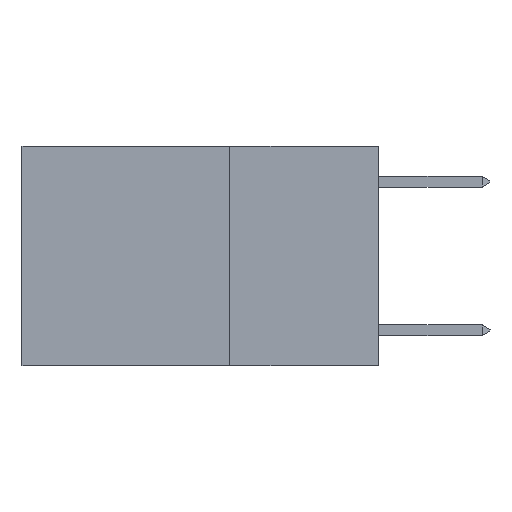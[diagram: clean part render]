
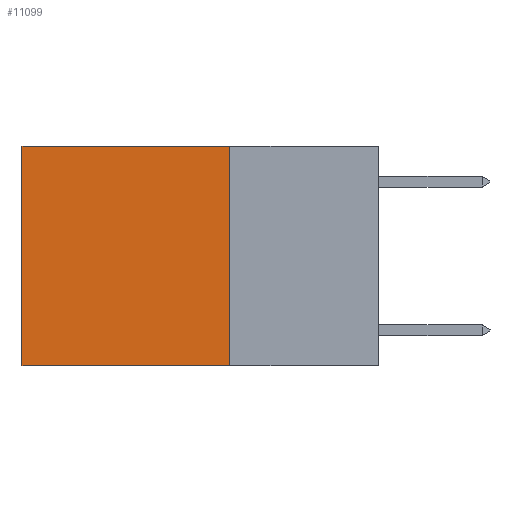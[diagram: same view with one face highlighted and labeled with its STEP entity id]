
A CAD part, left-side view. The second image highlights one B-rep face of the part: STEP entity #11099.
In plain terms, the highlighted planar face has unit normal (-1, 0, 0).
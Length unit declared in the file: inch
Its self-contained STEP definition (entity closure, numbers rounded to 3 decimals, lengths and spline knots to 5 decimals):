
#137 = EDGE_LOOP ( 'NONE', ( #4603, #12571, #2133, #2472 ) ) ;
#139 = CARTESIAN_POINT ( 'NONE',  ( 0.2625, 0.25, 0. ) ) ;
#140 = LINE ( 'NONE', #9520, #5739 ) ;
#470 = CARTESIAN_POINT ( 'NONE',  ( 0.2625, 0.6, 0. ) ) ;
#569 = FACE_OUTER_BOUND ( 'NONE', #137, .T. ) ;
#716 = EDGE_CURVE ( 'NONE', #3021, #2327, #140, .T. ) ;
#1998 = DIRECTION ( 'NONE',  ( 0., 0., -1. ) ) ;
#2043 = LINE ( 'NONE', #8048, #12786 ) ;
#2133 = ORIENTED_EDGE ( 'NONE', *, *, #7611, .F. ) ;
#2327 = VERTEX_POINT ( 'NONE', #470 ) ;
#2353 = CARTESIAN_POINT ( 'NONE',  ( 0.2625, 0.25, 0. ) ) ;
#2472 = ORIENTED_EDGE ( 'NONE', *, *, #716, .T. ) ;
#2477 = LINE ( 'NONE', #139, #12879 ) ;
#3000 = AXIS2_PLACEMENT_3D ( 'NONE', #2353, #12463, #6475 ) ;
#3021 = VERTEX_POINT ( 'NONE', #5981 ) ;
#3173 = EDGE_CURVE ( 'NONE', #2327, #10325, #10460, .T. ) ;
#3995 = EDGE_CURVE ( 'NONE', #10479, #10325, #2043, .T. ) ;
#4453 = PLANE ( 'NONE',  #3000 ) ;
#4603 = ORIENTED_EDGE ( 'NONE', *, *, #3173, .T. ) ;
#5022 = DIRECTION ( 'NONE',  ( 0., 1., 0. ) ) ;
#5739 = VECTOR ( 'NONE', #6524, 39.37008 ) ;
#5981 = CARTESIAN_POINT ( 'NONE',  ( 0.2625, 0.25, 0. ) ) ;
#6475 = DIRECTION ( 'NONE',  ( 0., 0., -1. ) ) ;
#6524 = DIRECTION ( 'NONE',  ( 0., 1., 0. ) ) ;
#6872 = CARTESIAN_POINT ( 'NONE',  ( 0.2625, 0.25, -0.37 ) ) ;
#7611 = EDGE_CURVE ( 'NONE', #3021, #10479, #2477, .T. ) ;
#8048 = CARTESIAN_POINT ( 'NONE',  ( 0.2625, 0.25, -0.37 ) ) ;
#9229 = CARTESIAN_POINT ( 'NONE',  ( 0.2625, 0.6, 0. ) ) ;
#9383 = DIRECTION ( 'NONE',  ( 0., 0., -1. ) ) ;
#9520 = CARTESIAN_POINT ( 'NONE',  ( 0.2625, 0.25, 0. ) ) ;
#10325 = VERTEX_POINT ( 'NONE', #11632 ) ;
#10460 = LINE ( 'NONE', #9229, #13106 ) ;
#10479 = VERTEX_POINT ( 'NONE', #6872 ) ;
#11099 = ADVANCED_FACE ( 'NONE', ( #569 ), #4453, .F. ) ;
#11632 = CARTESIAN_POINT ( 'NONE',  ( 0.2625, 0.6, -0.37 ) ) ;
#12463 = DIRECTION ( 'NONE',  ( 1., 0., 0. ) ) ;
#12571 = ORIENTED_EDGE ( 'NONE', *, *, #3995, .F. ) ;
#12786 = VECTOR ( 'NONE', #5022, 39.37008 ) ;
#12879 = VECTOR ( 'NONE', #9383, 39.37008 ) ;
#13106 = VECTOR ( 'NONE', #1998, 39.37008 ) ;
